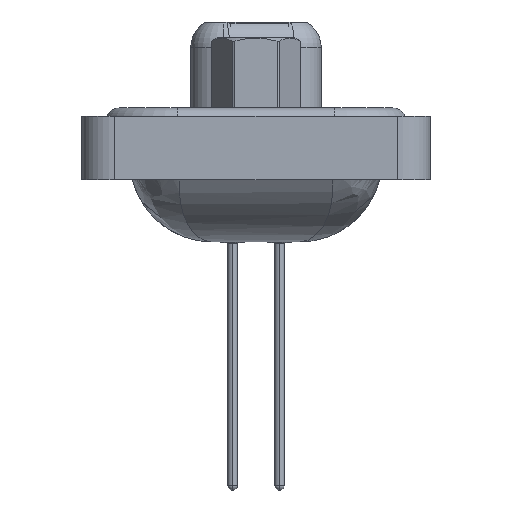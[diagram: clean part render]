
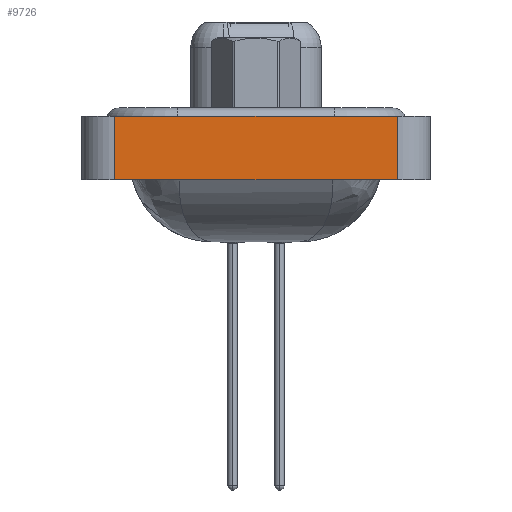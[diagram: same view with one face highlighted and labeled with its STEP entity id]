
A CAD part, left-side view. The second image highlights one B-rep face of the part: STEP entity #9726.
In plain terms, the highlighted planar face has unit normal (-1, 0, 0).
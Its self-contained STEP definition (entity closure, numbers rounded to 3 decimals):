
#402 = EDGE_CURVE ( 'NONE', #4522, #23171, #28266, .T. ) ;
#1403 = VECTOR ( 'NONE', #29059, 1000. ) ;
#2041 = LINE ( 'NONE', #13092, #1403 ) ;
#4522 = VERTEX_POINT ( 'NONE', #21247 ) ;
#5251 = EDGE_CURVE ( 'NONE', #28187, #4522, #2041, .T. ) ;
#5777 = CARTESIAN_POINT ( 'NONE',  ( -7.15, -8.55, -3.35 ) ) ;
#6112 = FACE_OUTER_BOUND ( 'NONE', #33953, .T. ) ;
#6837 = VECTOR ( 'NONE', #10088, 1000. ) ;
#8958 = CARTESIAN_POINT ( 'NONE',  ( -7.15, -8.55, -3.35 ) ) ;
#9653 = LINE ( 'NONE', #8958, #11776 ) ;
#9726 = ADVANCED_FACE ( 'NONE', ( #6112 ), #19116, .T. ) ;
#10042 = VECTOR ( 'NONE', #25282, 1000. ) ;
#10088 = DIRECTION ( 'NONE',  ( 0., -1., 0. ) ) ;
#10871 = AXIS2_PLACEMENT_3D ( 'NONE', #5777, #16512, #17030 ) ;
#11776 = VECTOR ( 'NONE', #20370, 1000. ) ;
#11950 = CARTESIAN_POINT ( 'NONE',  ( -7.15, -8.55, 0.5 ) ) ;
#13092 = CARTESIAN_POINT ( 'NONE',  ( -7.15, 8.55, -3.35 ) ) ;
#14102 = ORIENTED_EDGE ( 'NONE', *, *, #5251, .F. ) ;
#16512 = DIRECTION ( 'NONE',  ( -1., 0., 0. ) ) ;
#17030 = DIRECTION ( 'NONE',  ( 0., 0., 1. ) ) ;
#19116 = PLANE ( 'NONE',  #10871 ) ;
#20370 = DIRECTION ( 'NONE',  ( 0., 0., 1. ) ) ;
#21247 = CARTESIAN_POINT ( 'NONE',  ( -7.15, 8.55, 0.5 ) ) ;
#22893 = CARTESIAN_POINT ( 'NONE',  ( -7.15, -8.55, -3.35 ) ) ;
#23171 = VERTEX_POINT ( 'NONE', #26033 ) ;
#24153 = ORIENTED_EDGE ( 'NONE', *, *, #34655, .T. ) ;
#24213 = EDGE_CURVE ( 'NONE', #28187, #26748, #24845, .T. ) ;
#24845 = LINE ( 'NONE', #26401, #6837 ) ;
#25282 = DIRECTION ( 'NONE',  ( 0., -1., 0. ) ) ;
#26033 = CARTESIAN_POINT ( 'NONE',  ( -7.15, -8.55, 0.5 ) ) ;
#26401 = CARTESIAN_POINT ( 'NONE',  ( -7.15, -8.55, -3.35 ) ) ;
#26748 = VERTEX_POINT ( 'NONE', #22893 ) ;
#27935 = ORIENTED_EDGE ( 'NONE', *, *, #24213, .T. ) ;
#28187 = VERTEX_POINT ( 'NONE', #29449 ) ;
#28266 = LINE ( 'NONE', #11950, #10042 ) ;
#29059 = DIRECTION ( 'NONE',  ( 0., 0., 1. ) ) ;
#29449 = CARTESIAN_POINT ( 'NONE',  ( -7.15, 8.55, -3.35 ) ) ;
#31504 = ORIENTED_EDGE ( 'NONE', *, *, #402, .F. ) ;
#33953 = EDGE_LOOP ( 'NONE', ( #24153, #31504, #14102, #27935 ) ) ;
#34655 = EDGE_CURVE ( 'NONE', #26748, #23171, #9653, .T. ) ;
